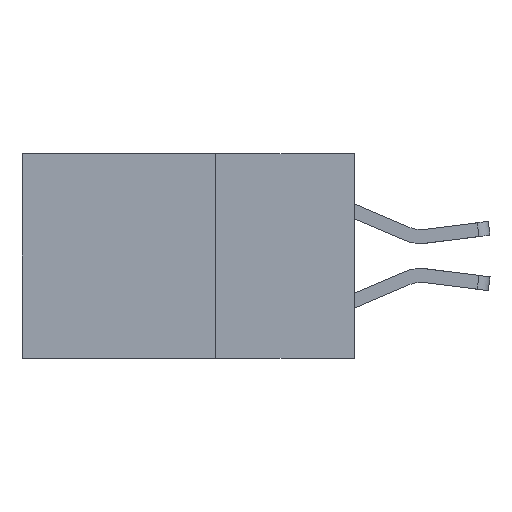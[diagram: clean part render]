
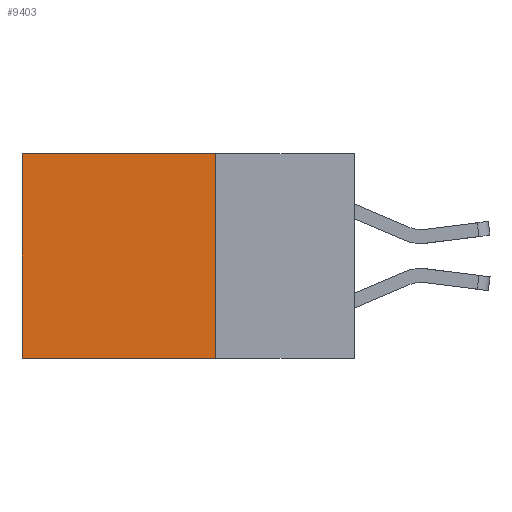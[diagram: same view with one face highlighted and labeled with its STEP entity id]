
A CAD part, left-side view. The second image highlights one B-rep face of the part: STEP entity #9403.
In plain terms, the highlighted planar face has unit normal (-1, 0, 0).
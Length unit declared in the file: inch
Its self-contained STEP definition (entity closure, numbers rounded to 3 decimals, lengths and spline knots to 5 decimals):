
#467 = EDGE_CURVE ( 'NONE', #2722, #10796, #1160, .T. ) ;
#550 = DIRECTION ( 'NONE',  ( 0., 1., 0. ) ) ;
#1029 = VECTOR ( 'NONE', #7792, 39.37008 ) ;
#1045 = VECTOR ( 'NONE', #6193, 39.37008 ) ;
#1138 = ORIENTED_EDGE ( 'NONE', *, *, #5228, .T. ) ;
#1153 = CARTESIAN_POINT ( 'NONE',  ( 0.298, 0.6, 0. ) ) ;
#1158 = CARTESIAN_POINT ( 'NONE',  ( 0.298, 0.25, -0.37 ) ) ;
#1160 = LINE ( 'NONE', #1158, #1045 ) ;
#1222 = ORIENTED_EDGE ( 'NONE', *, *, #467, .F. ) ;
#1644 = EDGE_CURVE ( 'NONE', #6014, #10796, #9290, .T. ) ;
#1681 = CARTESIAN_POINT ( 'NONE',  ( 0.298, 0.25, 0. ) ) ;
#1866 = CARTESIAN_POINT ( 'NONE',  ( 0.298, 0.6, -0.37 ) ) ;
#2722 = VERTEX_POINT ( 'NONE', #3063 ) ;
#3063 = CARTESIAN_POINT ( 'NONE',  ( 0.298, 0.25, -0.37 ) ) ;
#3663 = DIRECTION ( 'NONE',  ( 1., 0., 0. ) ) ;
#4376 = ORIENTED_EDGE ( 'NONE', *, *, #1644, .T. ) ;
#4399 = VECTOR ( 'NONE', #7547, 39.37008 ) ;
#4559 = FACE_OUTER_BOUND ( 'NONE', #8075, .T. ) ;
#4572 = EDGE_CURVE ( 'NONE', #7785, #2722, #9227, .T. ) ;
#4616 = CARTESIAN_POINT ( 'NONE',  ( 0.298, 0.25, 0. ) ) ;
#5228 = EDGE_CURVE ( 'NONE', #7785, #6014, #7644, .T. ) ;
#5448 = VECTOR ( 'NONE', #550, 39.37008 ) ;
#5498 = CARTESIAN_POINT ( 'NONE',  ( 0.298, 0.25, 0. ) ) ;
#6014 = VERTEX_POINT ( 'NONE', #1153 ) ;
#6193 = DIRECTION ( 'NONE',  ( 0., 1., 0. ) ) ;
#6219 = CARTESIAN_POINT ( 'NONE',  ( 0.298, 0.6, 0. ) ) ;
#6807 = AXIS2_PLACEMENT_3D ( 'NONE', #4616, #3663, #7939 ) ;
#7547 = DIRECTION ( 'NONE',  ( 0., 0., -1. ) ) ;
#7568 = CARTESIAN_POINT ( 'NONE',  ( 0.298, 0.25, 0. ) ) ;
#7644 = LINE ( 'NONE', #5498, #5448 ) ;
#7785 = VERTEX_POINT ( 'NONE', #7568 ) ;
#7792 = DIRECTION ( 'NONE',  ( 0., 0., -1. ) ) ;
#7939 = DIRECTION ( 'NONE',  ( 0., 0., -1. ) ) ;
#7948 = ORIENTED_EDGE ( 'NONE', *, *, #4572, .F. ) ;
#8075 = EDGE_LOOP ( 'NONE', ( #4376, #1222, #7948, #1138 ) ) ;
#9227 = LINE ( 'NONE', #1681, #4399 ) ;
#9290 = LINE ( 'NONE', #6219, #1029 ) ;
#9403 = ADVANCED_FACE ( 'NONE', ( #4559 ), #10302, .F. ) ;
#10302 = PLANE ( 'NONE',  #6807 ) ;
#10796 = VERTEX_POINT ( 'NONE', #1866 ) ;
